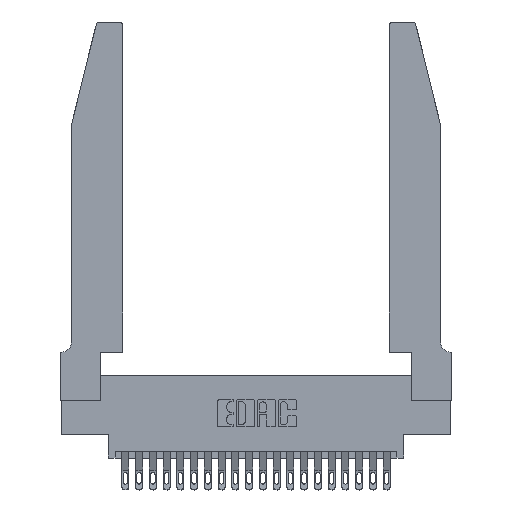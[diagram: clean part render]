
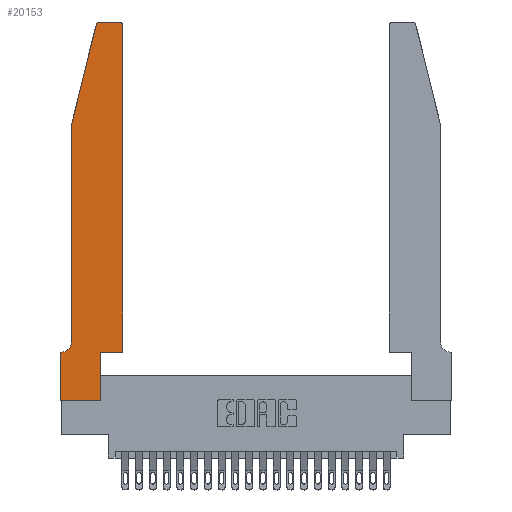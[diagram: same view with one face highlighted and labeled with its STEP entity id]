
A CAD part, top view. The second image highlights one B-rep face of the part: STEP entity #20153.
In plain terms, the highlighted planar face has unit normal (0, 0, 1).
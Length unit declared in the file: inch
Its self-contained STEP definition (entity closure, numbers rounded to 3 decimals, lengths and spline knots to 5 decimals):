
#31 = DIRECTION ( 'NONE',  ( 1., 0., 0. ) ) ;
#333 = VERTEX_POINT ( 'NONE', #8297 ) ;
#531 = VERTEX_POINT ( 'NONE', #12403 ) ;
#646 = VERTEX_POINT ( 'NONE', #14540 ) ;
#707 = EDGE_CURVE ( 'NONE', #333, #531, #20997, .T. ) ;
#853 = EDGE_CURVE ( 'NONE', #15749, #646, #2193, .T. ) ;
#1271 = CARTESIAN_POINT ( 'NONE',  ( 0.0755, 2., 0.37 ) ) ;
#1382 = CARTESIAN_POINT ( 'NONE',  ( 0., 0., 0.37 ) ) ;
#1574 = CARTESIAN_POINT ( 'NONE',  ( 0.4505, 0.35, 0.37 ) ) ;
#1944 = AXIS2_PLACEMENT_3D ( 'NONE', #6088, #13614, #2394 ) ;
#1956 = VECTOR ( 'NONE', #3007, 39.37008 ) ;
#2193 = LINE ( 'NONE', #14330, #11596 ) ;
#2394 = DIRECTION ( 'NONE',  ( 1., 0., 0. ) ) ;
#3007 = DIRECTION ( 'NONE',  ( -1., 0., 0. ) ) ;
#3215 = DIRECTION ( 'NONE',  ( 0., 1., 0. ) ) ;
#3237 = CARTESIAN_POINT ( 'NONE',  ( 0.0755, 2., 0.37 ) ) ;
#3881 = CARTESIAN_POINT ( 'NONE',  ( 0.0055, 0.42, 0.37 ) ) ;
#4465 = CIRCLE ( 'NONE', #12455, 0.07 ) ;
#4860 = VECTOR ( 'NONE', #21932, 39.37008 ) ;
#4914 = VECTOR ( 'NONE', #21861, 39.37008 ) ;
#4980 = EDGE_LOOP ( 'NONE', ( #8253, #12222, #6618, #19290, #15934, #16586, #14768, #16902, #5897, #20822, #6065, #8305 ) ) ;
#5392 = EDGE_CURVE ( 'NONE', #16642, #19399, #19613, .T. ) ;
#5758 = DIRECTION ( 'NONE',  ( -1., 0., 0. ) ) ;
#5763 = LINE ( 'NONE', #19696, #1956 ) ;
#5785 = VECTOR ( 'NONE', #18878, 39.37008 ) ;
#5841 = VERTEX_POINT ( 'NONE', #14858 ) ;
#5897 = ORIENTED_EDGE ( 'NONE', *, *, #16308, .T. ) ;
#6065 = ORIENTED_EDGE ( 'NONE', *, *, #13259, .T. ) ;
#6088 = CARTESIAN_POINT ( 'NONE',  ( 0., 0.35, 0.37 ) ) ;
#6512 = CARTESIAN_POINT ( 'NONE',  ( 0.25487, 2.72718, 0.37 ) ) ;
#6618 = ORIENTED_EDGE ( 'NONE', *, *, #8942, .T. ) ;
#7513 = CARTESIAN_POINT ( 'NONE',  ( 0.2605, 2.75, 0.37 ) ) ;
#8253 = ORIENTED_EDGE ( 'NONE', *, *, #14449, .T. ) ;
#8297 = CARTESIAN_POINT ( 'NONE',  ( 0.4505, 2.72, 0.37 ) ) ;
#8305 = ORIENTED_EDGE ( 'NONE', *, *, #707, .T. ) ;
#8392 = VECTOR ( 'NONE', #9395, 39.37008 ) ;
#8942 = EDGE_CURVE ( 'NONE', #12364, #15749, #21698, .T. ) ;
#9395 = DIRECTION ( 'NONE',  ( -1., 0., 0. ) ) ;
#9410 = CARTESIAN_POINT ( 'NONE',  ( 0.284, 2.75, 0.37 ) ) ;
#9614 = EDGE_CURVE ( 'NONE', #5841, #23539, #18298, .T. ) ;
#10616 = CARTESIAN_POINT ( 'NONE',  ( 0.2865, 0., 0.37 ) ) ;
#11049 = CARTESIAN_POINT ( 'NONE',  ( 0.4505, 0.35, 0.37 ) ) ;
#11229 = DIRECTION ( 'NONE',  ( 0., 0., 1. ) ) ;
#11596 = VECTOR ( 'NONE', #12782, 39.37008 ) ;
#11758 = PLANE ( 'NONE',  #1944 ) ;
#12222 = ORIENTED_EDGE ( 'NONE', *, *, #23238, .T. ) ;
#12364 = VERTEX_POINT ( 'NONE', #6512 ) ;
#12403 = CARTESIAN_POINT ( 'NONE',  ( 0.4205, 2.75, 0.37 ) ) ;
#12419 = CARTESIAN_POINT ( 'NONE',  ( 0., 0., 0.37 ) ) ;
#12455 = AXIS2_PLACEMENT_3D ( 'NONE', #3881, #16891, #5758 ) ;
#12782 = DIRECTION ( 'NONE',  ( 0., -1., 0. ) ) ;
#12915 = VERTEX_POINT ( 'NONE', #10616 ) ;
#13059 = EDGE_CURVE ( 'NONE', #23539, #12915, #14837, .T. ) ;
#13147 = AXIS2_PLACEMENT_3D ( 'NONE', #22132, #11229, #31 ) ;
#13259 = EDGE_CURVE ( 'NONE', #19399, #333, #15692, .T. ) ;
#13595 = CARTESIAN_POINT ( 'NONE',  ( 0.2865, 0.35, 0.37 ) ) ;
#13614 = DIRECTION ( 'NONE',  ( 0., 0., 1. ) ) ;
#14327 = DIRECTION ( 'NONE',  ( -0.239, -0.971, 0. ) ) ;
#14330 = CARTESIAN_POINT ( 'NONE',  ( 0.0755, 2., 0.37 ) ) ;
#14449 = EDGE_CURVE ( 'NONE', #531, #15287, #18228, .T. ) ;
#14540 = CARTESIAN_POINT ( 'NONE',  ( 0.0755, 0.42, 0.37 ) ) ;
#14644 = CARTESIAN_POINT ( 'NONE',  ( 0., 0., 0.37 ) ) ;
#14768 = ORIENTED_EDGE ( 'NONE', *, *, #9614, .T. ) ;
#14837 = LINE ( 'NONE', #14644, #4914 ) ;
#14858 = CARTESIAN_POINT ( 'NONE',  ( 0., 0.35, 0.37 ) ) ;
#15287 = VERTEX_POINT ( 'NONE', #9410 ) ;
#15590 = CARTESIAN_POINT ( 'NONE',  ( 0.0055, 0.35, 0.37 ) ) ;
#15692 = LINE ( 'NONE', #20672, #5785 ) ;
#15749 = VERTEX_POINT ( 'NONE', #3237 ) ;
#15934 = ORIENTED_EDGE ( 'NONE', *, *, #20011, .T. ) ;
#16155 = VECTOR ( 'NONE', #3215, 39.37008 ) ;
#16247 = CARTESIAN_POINT ( 'NONE',  ( 0.2865, 0.35, 0.37 ) ) ;
#16308 = EDGE_CURVE ( 'NONE', #12915, #16642, #23512, .T. ) ;
#16586 = ORIENTED_EDGE ( 'NONE', *, *, #22982, .T. ) ;
#16642 = VERTEX_POINT ( 'NONE', #13595 ) ;
#16891 = DIRECTION ( 'NONE',  ( 0., 0., -1. ) ) ;
#16902 = ORIENTED_EDGE ( 'NONE', *, *, #13059, .T. ) ;
#18228 = LINE ( 'NONE', #7513, #8392 ) ;
#18298 = LINE ( 'NONE', #1382, #22538 ) ;
#18878 = DIRECTION ( 'NONE',  ( 0., 1., 0. ) ) ;
#19290 = ORIENTED_EDGE ( 'NONE', *, *, #853, .T. ) ;
#19399 = VERTEX_POINT ( 'NONE', #11049 ) ;
#19484 = FACE_OUTER_BOUND ( 'NONE', #4980, .T. ) ;
#19613 = LINE ( 'NONE', #1574, #4860 ) ;
#19696 = CARTESIAN_POINT ( 'NONE',  ( 0.0755, 0.35, 0.37 ) ) ;
#19812 = DIRECTION ( 'NONE',  ( 0., 0., 1. ) ) ;
#20011 = EDGE_CURVE ( 'NONE', #646, #22866, #4465, .T. ) ;
#20153 = ADVANCED_FACE ( 'NONE', ( #19484 ), #11758, .T. ) ;
#20190 = CIRCLE ( 'NONE', #13147, 0.03 ) ;
#20672 = CARTESIAN_POINT ( 'NONE',  ( 0.4505, 0.35, 0.37 ) ) ;
#20822 = ORIENTED_EDGE ( 'NONE', *, *, #5392, .T. ) ;
#20997 = CIRCLE ( 'NONE', #22374, 0.03 ) ;
#21698 = LINE ( 'NONE', #1271, #22843 ) ;
#21735 = DIRECTION ( 'NONE',  ( 0., -1., 0. ) ) ;
#21861 = DIRECTION ( 'NONE',  ( 1., 0., 0. ) ) ;
#21932 = DIRECTION ( 'NONE',  ( 1., 0., 0. ) ) ;
#22132 = CARTESIAN_POINT ( 'NONE',  ( 0.284, 2.72, 0.37 ) ) ;
#22245 = DIRECTION ( 'NONE',  ( 1., 0., 0. ) ) ;
#22374 = AXIS2_PLACEMENT_3D ( 'NONE', #23446, #19812, #22245 ) ;
#22538 = VECTOR ( 'NONE', #21735, 39.37008 ) ;
#22843 = VECTOR ( 'NONE', #14327, 39.37008 ) ;
#22866 = VERTEX_POINT ( 'NONE', #15590 ) ;
#22982 = EDGE_CURVE ( 'NONE', #22866, #5841, #5763, .T. ) ;
#23238 = EDGE_CURVE ( 'NONE', #15287, #12364, #20190, .T. ) ;
#23446 = CARTESIAN_POINT ( 'NONE',  ( 0.4205, 2.72, 0.37 ) ) ;
#23512 = LINE ( 'NONE', #16247, #16155 ) ;
#23539 = VERTEX_POINT ( 'NONE', #12419 ) ;
